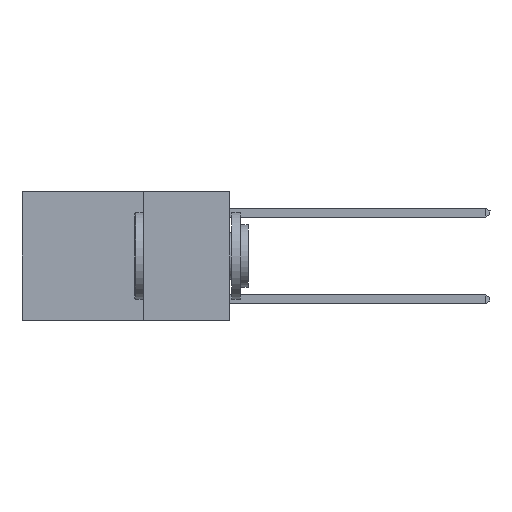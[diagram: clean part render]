
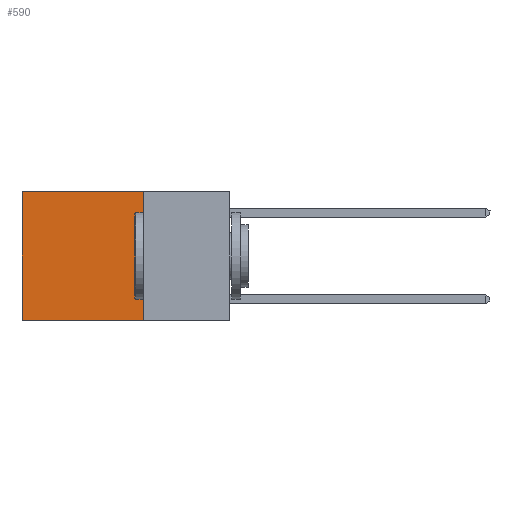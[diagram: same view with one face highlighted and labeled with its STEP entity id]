
A CAD part, left-side view. The second image highlights one B-rep face of the part: STEP entity #590.
In plain terms, the highlighted planar face has unit normal (-1, 0, 0).
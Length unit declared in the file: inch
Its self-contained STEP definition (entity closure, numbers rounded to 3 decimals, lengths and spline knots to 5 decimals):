
#152 = DIRECTION ( 'NONE',  ( 0., 1., 0. ) ) ;
#590 = ADVANCED_FACE ( 'NONE', ( #6635 ), #17733, .F. ) ;
#1011 = VECTOR ( 'NONE', #152, 39.37008 ) ;
#1746 = ORIENTED_EDGE ( 'NONE', *, *, #9393, .T. ) ;
#1803 = VECTOR ( 'NONE', #4622, 39.37008 ) ;
#3160 = CARTESIAN_POINT ( 'NONE',  ( 0.2625, 0.25, -0.37 ) ) ;
#3920 = VERTEX_POINT ( 'NONE', #19686 ) ;
#4622 = DIRECTION ( 'NONE',  ( 0., 1., 0. ) ) ;
#5027 = CARTESIAN_POINT ( 'NONE',  ( 0.2625, 0.25, 0. ) ) ;
#5631 = LINE ( 'NONE', #15940, #1803 ) ;
#6303 = AXIS2_PLACEMENT_3D ( 'NONE', #5027, #8250, #16454 ) ;
#6544 = DIRECTION ( 'NONE',  ( 0., 0., -1. ) ) ;
#6635 = FACE_OUTER_BOUND ( 'NONE', #7770, .T. ) ;
#7770 = EDGE_LOOP ( 'NONE', ( #12760, #15267, #20032, #1746 ) ) ;
#8248 = EDGE_CURVE ( 'NONE', #3920, #12546, #19795, .T. ) ;
#8250 = DIRECTION ( 'NONE',  ( 1., 0., 0. ) ) ;
#9393 = EDGE_CURVE ( 'NONE', #3920, #19013, #5631, .T. ) ;
#9618 = VECTOR ( 'NONE', #6544, 39.37008 ) ;
#9770 = VERTEX_POINT ( 'NONE', #18400 ) ;
#10774 = LINE ( 'NONE', #16354, #19731 ) ;
#11840 = CARTESIAN_POINT ( 'NONE',  ( 0.2625, 0.6, 0. ) ) ;
#12546 = VERTEX_POINT ( 'NONE', #15325 ) ;
#12728 = EDGE_CURVE ( 'NONE', #19013, #9770, #10774, .T. ) ;
#12760 = ORIENTED_EDGE ( 'NONE', *, *, #12728, .T. ) ;
#15189 = EDGE_CURVE ( 'NONE', #12546, #9770, #16628, .T. ) ;
#15267 = ORIENTED_EDGE ( 'NONE', *, *, #15189, .F. ) ;
#15325 = CARTESIAN_POINT ( 'NONE',  ( 0.2625, 0.25, -0.37 ) ) ;
#15940 = CARTESIAN_POINT ( 'NONE',  ( 0.2625, 0.25, 0. ) ) ;
#16354 = CARTESIAN_POINT ( 'NONE',  ( 0.2625, 0.6, 0. ) ) ;
#16454 = DIRECTION ( 'NONE',  ( 0., 0., -1. ) ) ;
#16628 = LINE ( 'NONE', #3160, #1011 ) ;
#17733 = PLANE ( 'NONE',  #6303 ) ;
#17969 = CARTESIAN_POINT ( 'NONE',  ( 0.2625, 0.25, 0. ) ) ;
#18400 = CARTESIAN_POINT ( 'NONE',  ( 0.2625, 0.6, -0.37 ) ) ;
#19013 = VERTEX_POINT ( 'NONE', #11840 ) ;
#19068 = DIRECTION ( 'NONE',  ( 0., 0., -1. ) ) ;
#19686 = CARTESIAN_POINT ( 'NONE',  ( 0.2625, 0.25, 0. ) ) ;
#19731 = VECTOR ( 'NONE', #19068, 39.37008 ) ;
#19795 = LINE ( 'NONE', #17969, #9618 ) ;
#20032 = ORIENTED_EDGE ( 'NONE', *, *, #8248, .F. ) ;
